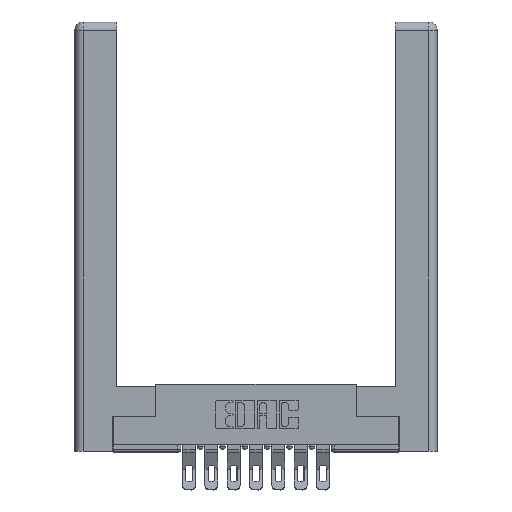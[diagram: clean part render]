
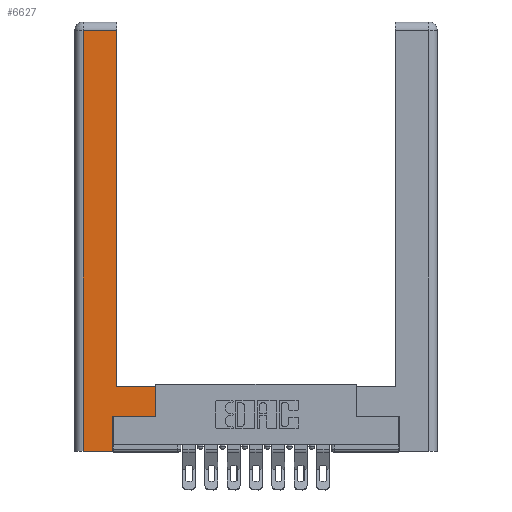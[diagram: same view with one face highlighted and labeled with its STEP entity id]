
A CAD part, top view. The second image highlights one B-rep face of the part: STEP entity #6627.
In plain terms, the highlighted planar face has unit normal (0, 0, 1).
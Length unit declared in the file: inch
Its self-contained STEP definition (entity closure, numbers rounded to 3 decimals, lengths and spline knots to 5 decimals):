
#76 = DIRECTION ( 'NONE',  ( 0., 1., 0. ) ) ;
#104 = EDGE_LOOP ( 'NONE', ( #4338, #3420, #1744, #311, #1896, #12126, #6741, #5516 ) ) ;
#311 = ORIENTED_EDGE ( 'NONE', *, *, #10568, .T. ) ;
#1404 = LINE ( 'NONE', #12131, #9394 ) ;
#1744 = ORIENTED_EDGE ( 'NONE', *, *, #12554, .T. ) ;
#1896 = ORIENTED_EDGE ( 'NONE', *, *, #2684, .T. ) ;
#2032 = VERTEX_POINT ( 'NONE', #6447 ) ;
#2238 = VERTEX_POINT ( 'NONE', #13245 ) ;
#2684 = EDGE_CURVE ( 'NONE', #7060, #11870, #9852, .T. ) ;
#2773 = DIRECTION ( 'NONE',  ( -1., 0., 0. ) ) ;
#2913 = DIRECTION ( 'NONE',  ( 0., 1., 0. ) ) ;
#3351 = CARTESIAN_POINT ( 'NONE',  ( 0.295, 0.45, 0. ) ) ;
#3420 = ORIENTED_EDGE ( 'NONE', *, *, #10094, .T. ) ;
#3725 = CARTESIAN_POINT ( 'NONE',  ( 0.265, 0., 0. ) ) ;
#3924 = CARTESIAN_POINT ( 'NONE',  ( 0.0615, 2.94, 0. ) ) ;
#3940 = CARTESIAN_POINT ( 'NONE',  ( 0.565, 0.45, 0. ) ) ;
#4116 = LINE ( 'NONE', #8262, #13581 ) ;
#4338 = ORIENTED_EDGE ( 'NONE', *, *, #4965, .T. ) ;
#4537 = DIRECTION ( 'NONE',  ( -1., 0., 0. ) ) ;
#4636 = EDGE_CURVE ( 'NONE', #10989, #6526, #1404, .T. ) ;
#4790 = DIRECTION ( 'NONE',  ( 0., 0., -1. ) ) ;
#4965 = EDGE_CURVE ( 'NONE', #6526, #8917, #11506, .T. ) ;
#5165 = CARTESIAN_POINT ( 'NONE',  ( 0.295, 2.94, 0. ) ) ;
#5203 = CARTESIAN_POINT ( 'NONE',  ( 0.565, 0.245, 0. ) ) ;
#5516 = ORIENTED_EDGE ( 'NONE', *, *, #4636, .T. ) ;
#5869 = CARTESIAN_POINT ( 'NONE',  ( 0.565, 0.45, 0. ) ) ;
#6321 = VECTOR ( 'NONE', #76, 39.37008 ) ;
#6447 = CARTESIAN_POINT ( 'NONE',  ( 0.0615, 0., 0. ) ) ;
#6526 = VERTEX_POINT ( 'NONE', #3351 ) ;
#6627 = ADVANCED_FACE ( 'NONE', ( #6736 ), #7974, .F. ) ;
#6736 = FACE_OUTER_BOUND ( 'NONE', #104, .T. ) ;
#6741 = ORIENTED_EDGE ( 'NONE', *, *, #11197, .T. ) ;
#6840 = CARTESIAN_POINT ( 'NONE',  ( 0.0615, 0., 0. ) ) ;
#7060 = VERTEX_POINT ( 'NONE', #3725 ) ;
#7419 = DIRECTION ( 'NONE',  ( 1., 0., 0. ) ) ;
#7943 = LINE ( 'NONE', #6840, #10253 ) ;
#7974 = PLANE ( 'NONE',  #10985 ) ;
#8262 = CARTESIAN_POINT ( 'NONE',  ( 0.565, 0.245, 0. ) ) ;
#8470 = CARTESIAN_POINT ( 'NONE',  ( 0.265, 0.245, 0. ) ) ;
#8870 = VECTOR ( 'NONE', #2773, 39.37008 ) ;
#8917 = VERTEX_POINT ( 'NONE', #5165 ) ;
#9045 = LINE ( 'NONE', #5869, #12046 ) ;
#9394 = VECTOR ( 'NONE', #4537, 39.37008 ) ;
#9852 = LINE ( 'NONE', #12288, #13517 ) ;
#10094 = EDGE_CURVE ( 'NONE', #8917, #2238, #13436, .T. ) ;
#10110 = DIRECTION ( 'NONE',  ( 0., 1., 0. ) ) ;
#10253 = VECTOR ( 'NONE', #13099, 39.37008 ) ;
#10358 = CARTESIAN_POINT ( 'NONE',  ( 0.265, 0., 0. ) ) ;
#10458 = VERTEX_POINT ( 'NONE', #5203 ) ;
#10568 = EDGE_CURVE ( 'NONE', #2032, #7060, #11496, .T. ) ;
#10985 = AXIS2_PLACEMENT_3D ( 'NONE', #11081, #4790, #13262 ) ;
#10989 = VERTEX_POINT ( 'NONE', #3940 ) ;
#11081 = CARTESIAN_POINT ( 'NONE',  ( 0., 0., 0. ) ) ;
#11197 = EDGE_CURVE ( 'NONE', #10458, #10989, #9045, .T. ) ;
#11449 = DIRECTION ( 'NONE',  ( 1., 0., 0. ) ) ;
#11496 = LINE ( 'NONE', #10358, #13107 ) ;
#11506 = LINE ( 'NONE', #11651, #6321 ) ;
#11651 = CARTESIAN_POINT ( 'NONE',  ( 0.295, 3., 0. ) ) ;
#11728 = EDGE_CURVE ( 'NONE', #11870, #10458, #4116, .T. ) ;
#11870 = VERTEX_POINT ( 'NONE', #8470 ) ;
#12046 = VECTOR ( 'NONE', #10110, 39.37008 ) ;
#12126 = ORIENTED_EDGE ( 'NONE', *, *, #11728, .T. ) ;
#12131 = CARTESIAN_POINT ( 'NONE',  ( 0.295, 0.45, 0. ) ) ;
#12288 = CARTESIAN_POINT ( 'NONE',  ( 0.265, 0.245, 0. ) ) ;
#12554 = EDGE_CURVE ( 'NONE', #2238, #2032, #7943, .T. ) ;
#13099 = DIRECTION ( 'NONE',  ( 0., -1., 0. ) ) ;
#13107 = VECTOR ( 'NONE', #7419, 39.37008 ) ;
#13245 = CARTESIAN_POINT ( 'NONE',  ( 0.0615, 2.94, 0. ) ) ;
#13262 = DIRECTION ( 'NONE',  ( -1., 0., 0. ) ) ;
#13436 = LINE ( 'NONE', #3924, #8870 ) ;
#13517 = VECTOR ( 'NONE', #2913, 39.37008 ) ;
#13581 = VECTOR ( 'NONE', #11449, 39.37008 ) ;
